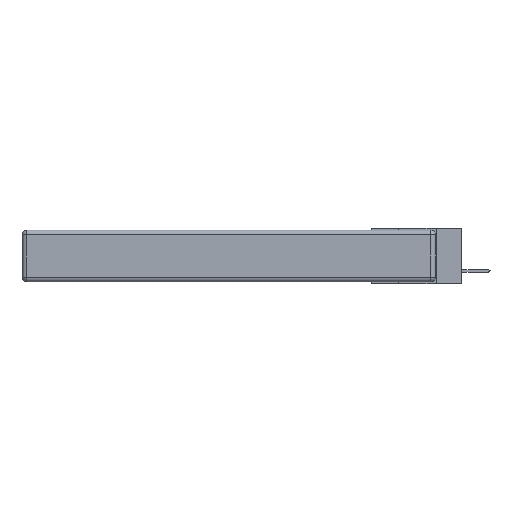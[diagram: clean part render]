
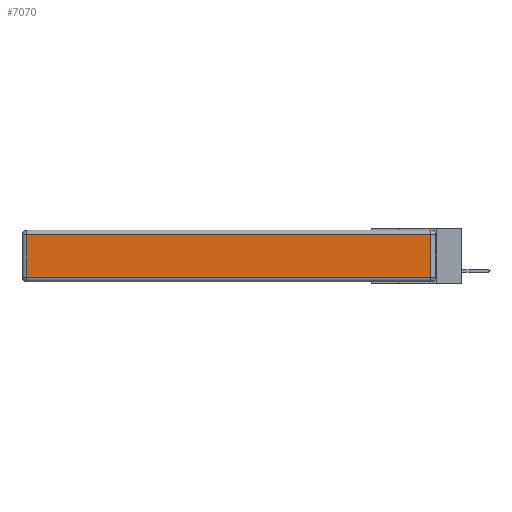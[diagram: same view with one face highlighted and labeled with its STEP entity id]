
A CAD part, left-side view. The second image highlights one B-rep face of the part: STEP entity #7070.
In plain terms, the highlighted planar face has unit normal (-1, 0, 0).
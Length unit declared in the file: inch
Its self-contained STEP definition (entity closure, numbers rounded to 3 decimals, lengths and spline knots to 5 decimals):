
#314 = ORIENTED_EDGE ( 'NONE', *, *, #11776, .T. ) ;
#382 = VECTOR ( 'NONE', #8520, 39.37008 ) ;
#808 = DIRECTION ( 'NONE',  ( -1., 0., 0. ) ) ;
#991 = CARTESIAN_POINT ( 'NONE',  ( 0., 2.75, -0.03 ) ) ;
#1247 = CARTESIAN_POINT ( 'NONE',  ( 0., 2.72, -0.343 ) ) ;
#1376 = DIRECTION ( 'NONE',  ( 0., 0., 1. ) ) ;
#1787 = FACE_OUTER_BOUND ( 'NONE', #10725, .T. ) ;
#1886 = VERTEX_POINT ( 'NONE', #10013 ) ;
#3065 = CARTESIAN_POINT ( 'NONE',  ( 0., 0.03, -0.343 ) ) ;
#3731 = VECTOR ( 'NONE', #9085, 39.37008 ) ;
#3755 = ORIENTED_EDGE ( 'NONE', *, *, #6999, .T. ) ;
#4344 = ORIENTED_EDGE ( 'NONE', *, *, #6257, .T. ) ;
#4498 = CARTESIAN_POINT ( 'NONE',  ( 0., 2.72, -0.313 ) ) ;
#4775 = AXIS2_PLACEMENT_3D ( 'NONE', #8298, #808, #12079 ) ;
#5495 = LINE ( 'NONE', #3065, #6683 ) ;
#5585 = CARTESIAN_POINT ( 'NONE',  ( 0., 0., -0.313 ) ) ;
#5613 = VECTOR ( 'NONE', #7528, 39.37008 ) ;
#6244 = LINE ( 'NONE', #1247, #3731 ) ;
#6257 = EDGE_CURVE ( 'NONE', #1886, #9683, #8008, .T. ) ;
#6683 = VECTOR ( 'NONE', #1376, 39.37008 ) ;
#6910 = EDGE_CURVE ( 'NONE', #9683, #11627, #6244, .T. ) ;
#6999 = EDGE_CURVE ( 'NONE', #11529, #1886, #5495, .T. ) ;
#7070 = ADVANCED_FACE ( 'NONE', ( #1787 ), #7367, .T. ) ;
#7367 = PLANE ( 'NONE',  #4775 ) ;
#7528 = DIRECTION ( 'NONE',  ( 0., -1., 0. ) ) ;
#8008 = LINE ( 'NONE', #991, #382 ) ;
#8298 = CARTESIAN_POINT ( 'NONE',  ( 0., 0., -0.343 ) ) ;
#8520 = DIRECTION ( 'NONE',  ( 0., 1., 0. ) ) ;
#9080 = CARTESIAN_POINT ( 'NONE',  ( 0., 0.03, -0.313 ) ) ;
#9085 = DIRECTION ( 'NONE',  ( 0., 0., -1. ) ) ;
#9683 = VERTEX_POINT ( 'NONE', #11017 ) ;
#10013 = CARTESIAN_POINT ( 'NONE',  ( 0., 0.03, -0.03 ) ) ;
#10024 = LINE ( 'NONE', #5585, #5613 ) ;
#10725 = EDGE_LOOP ( 'NONE', ( #314, #3755, #4344, #11752 ) ) ;
#11017 = CARTESIAN_POINT ( 'NONE',  ( 0., 2.72, -0.03 ) ) ;
#11529 = VERTEX_POINT ( 'NONE', #9080 ) ;
#11627 = VERTEX_POINT ( 'NONE', #4498 ) ;
#11752 = ORIENTED_EDGE ( 'NONE', *, *, #6910, .T. ) ;
#11776 = EDGE_CURVE ( 'NONE', #11627, #11529, #10024, .T. ) ;
#12079 = DIRECTION ( 'NONE',  ( 0., 0., 1. ) ) ;
